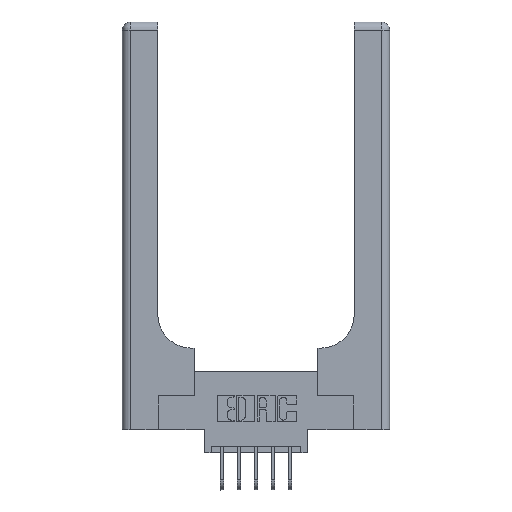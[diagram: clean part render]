
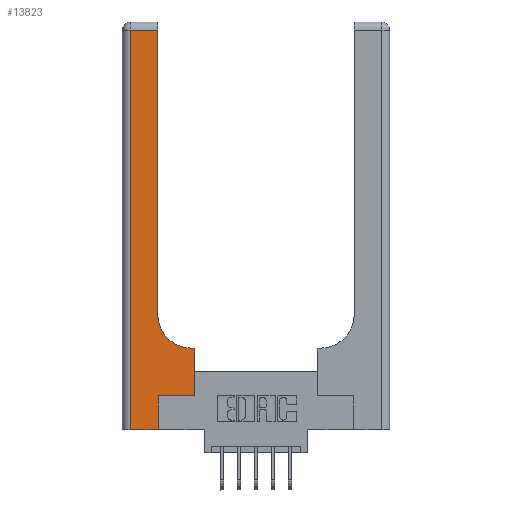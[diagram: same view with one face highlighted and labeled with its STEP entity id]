
A CAD part, top view. The second image highlights one B-rep face of the part: STEP entity #13823.
In plain terms, the highlighted planar face has unit normal (0, 0, 1).
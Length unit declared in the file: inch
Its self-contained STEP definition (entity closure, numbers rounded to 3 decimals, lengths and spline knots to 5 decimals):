
#34 = CARTESIAN_POINT ( 'NONE',  ( 0.26, 3., 0.37 ) ) ;
#296 = EDGE_CURVE ( 'NONE', #2007, #8035, #7548, .T. ) ;
#506 = PLANE ( 'NONE',  #9022 ) ;
#990 = LINE ( 'NONE', #11400, #10289 ) ;
#1416 = LINE ( 'NONE', #2649, #6147 ) ;
#1642 = ORIENTED_EDGE ( 'NONE', *, *, #11636, .T. ) ;
#1741 = DIRECTION ( 'NONE',  ( 0., 0., -1. ) ) ;
#1757 = ORIENTED_EDGE ( 'NONE', *, *, #9967, .T. ) ;
#1848 = LINE ( 'NONE', #13145, #14080 ) ;
#2007 = VERTEX_POINT ( 'NONE', #2619 ) ;
#2164 = LINE ( 'NONE', #5752, #12920 ) ;
#2251 = CARTESIAN_POINT ( 'NONE',  ( 0.265, 0., 0.37 ) ) ;
#2287 = CARTESIAN_POINT ( 'NONE',  ( 0.265, 0.25, 0.37 ) ) ;
#2619 = CARTESIAN_POINT ( 'NONE',  ( 0.528, 0.6, 0.37 ) ) ;
#2622 = FACE_OUTER_BOUND ( 'NONE', #3227, .T. ) ;
#2642 = DIRECTION ( 'NONE',  ( 0., 0., -1. ) ) ;
#2649 = CARTESIAN_POINT ( 'NONE',  ( 0., 2.94, 0.37 ) ) ;
#2985 = CARTESIAN_POINT ( 'NONE',  ( 0.51, 0.6, 0.37 ) ) ;
#3098 = EDGE_CURVE ( 'NONE', #5329, #8522, #990, .T. ) ;
#3177 = DIRECTION ( 'NONE',  ( 1., 0., 0. ) ) ;
#3227 = EDGE_LOOP ( 'NONE', ( #1757, #1642, #14200, #5521, #10582, #15286, #9734, #15061, #8791 ) ) ;
#3793 = EDGE_CURVE ( 'NONE', #11575, #6733, #2164, .T. ) ;
#3950 = VECTOR ( 'NONE', #7151, 39.37008 ) ;
#4723 = EDGE_CURVE ( 'NONE', #6733, #12735, #13394, .T. ) ;
#4952 = DIRECTION ( 'NONE',  ( -1., 0., 0. ) ) ;
#5191 = VERTEX_POINT ( 'NONE', #5799 ) ;
#5329 = VERTEX_POINT ( 'NONE', #2287 ) ;
#5491 = VECTOR ( 'NONE', #14431, 39.37008 ) ;
#5495 = EDGE_CURVE ( 'NONE', #8035, #5581, #10670, .T. ) ;
#5521 = ORIENTED_EDGE ( 'NONE', *, *, #4723, .T. ) ;
#5581 = VERTEX_POINT ( 'NONE', #9608 ) ;
#5752 = CARTESIAN_POINT ( 'NONE',  ( 0.06, 3., 0.37 ) ) ;
#5799 = CARTESIAN_POINT ( 'NONE',  ( 0.26, 2.94, 0.37 ) ) ;
#5863 = CARTESIAN_POINT ( 'NONE',  ( 0.528, 0.25, 0.37 ) ) ;
#6020 = LINE ( 'NONE', #34, #8621 ) ;
#6081 = DIRECTION ( 'NONE',  ( 0., 1., 0. ) ) ;
#6147 = VECTOR ( 'NONE', #4952, 39.37008 ) ;
#6733 = VERTEX_POINT ( 'NONE', #12534 ) ;
#6822 = DIRECTION ( 'NONE',  ( 0., -1., 0. ) ) ;
#6930 = CARTESIAN_POINT ( 'NONE',  ( 0.26, 0.6, 0.37 ) ) ;
#7151 = DIRECTION ( 'NONE',  ( 0., 1., 0. ) ) ;
#7548 = LINE ( 'NONE', #6930, #8295 ) ;
#8035 = VERTEX_POINT ( 'NONE', #2985 ) ;
#8183 = DIRECTION ( 'NONE',  ( -1., 0., 0. ) ) ;
#8295 = VECTOR ( 'NONE', #8183, 39.37008 ) ;
#8448 = EDGE_CURVE ( 'NONE', #12735, #5329, #1848, .T. ) ;
#8522 = VERTEX_POINT ( 'NONE', #9972 ) ;
#8621 = VECTOR ( 'NONE', #6081, 39.37008 ) ;
#8788 = CARTESIAN_POINT ( 'NONE',  ( 0., 0., 0.37 ) ) ;
#8791 = ORIENTED_EDGE ( 'NONE', *, *, #5495, .T. ) ;
#8855 = DIRECTION ( 'NONE',  ( -1., 0., 0. ) ) ;
#9022 = AXIS2_PLACEMENT_3D ( 'NONE', #11257, #1741, #8855 ) ;
#9485 = DIRECTION ( 'NONE',  ( 0., 1., 0. ) ) ;
#9608 = CARTESIAN_POINT ( 'NONE',  ( 0.26, 0.85, 0.37 ) ) ;
#9734 = ORIENTED_EDGE ( 'NONE', *, *, #13591, .T. ) ;
#9862 = LINE ( 'NONE', #5863, #3950 ) ;
#9967 = EDGE_CURVE ( 'NONE', #5581, #5191, #6020, .T. ) ;
#9972 = CARTESIAN_POINT ( 'NONE',  ( 0.528, 0.25, 0.37 ) ) ;
#10289 = VECTOR ( 'NONE', #3177, 39.37008 ) ;
#10582 = ORIENTED_EDGE ( 'NONE', *, *, #8448, .T. ) ;
#10670 = CIRCLE ( 'NONE', #14828, 0.25 ) ;
#10808 = CARTESIAN_POINT ( 'NONE',  ( 0.51, 0.85, 0.37 ) ) ;
#11257 = CARTESIAN_POINT ( 'NONE',  ( 0., 3., 0.37 ) ) ;
#11400 = CARTESIAN_POINT ( 'NONE',  ( 0.265, 0.25, 0.37 ) ) ;
#11575 = VERTEX_POINT ( 'NONE', #13002 ) ;
#11636 = EDGE_CURVE ( 'NONE', #5191, #11575, #1416, .T. ) ;
#12534 = CARTESIAN_POINT ( 'NONE',  ( 0.06, 0., 0.37 ) ) ;
#12735 = VERTEX_POINT ( 'NONE', #2251 ) ;
#12920 = VECTOR ( 'NONE', #6822, 39.37008 ) ;
#13002 = CARTESIAN_POINT ( 'NONE',  ( 0.06, 2.94, 0.37 ) ) ;
#13145 = CARTESIAN_POINT ( 'NONE',  ( 0.265, 0., 0.37 ) ) ;
#13394 = LINE ( 'NONE', #8788, #5491 ) ;
#13591 = EDGE_CURVE ( 'NONE', #8522, #2007, #9862, .T. ) ;
#13823 = ADVANCED_FACE ( 'NONE', ( #2622 ), #506, .F. ) ;
#14080 = VECTOR ( 'NONE', #9485, 39.37008 ) ;
#14200 = ORIENTED_EDGE ( 'NONE', *, *, #3793, .T. ) ;
#14424 = DIRECTION ( 'NONE',  ( 1., 0., 0. ) ) ;
#14431 = DIRECTION ( 'NONE',  ( 1., 0., 0. ) ) ;
#14828 = AXIS2_PLACEMENT_3D ( 'NONE', #10808, #2642, #14424 ) ;
#15061 = ORIENTED_EDGE ( 'NONE', *, *, #296, .T. ) ;
#15286 = ORIENTED_EDGE ( 'NONE', *, *, #3098, .T. ) ;
